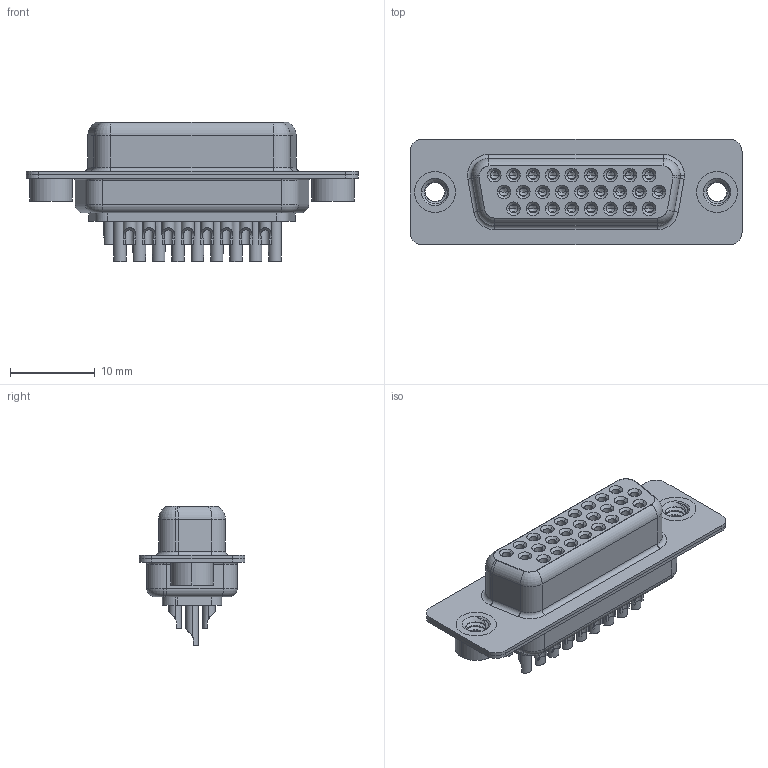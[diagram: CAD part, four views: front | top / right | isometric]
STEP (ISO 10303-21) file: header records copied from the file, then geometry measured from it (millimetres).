
FILE_DESCRIPTION (( 'STEP AP203' ), '1' );
FILE_NAME ('638-M26-332-BN2.STEP', '2022-07-05T19:32:56', ( '' ), ( '' ), 'SwSTEP 2.0', 'SolidWorks 2020', '' );
FILE_SCHEMA (( 'CONFIG_CONTROL_DESIGN' ));
Length unit declared in the file: millimetre
Products named in the file (8): 638M Shell Rear_26 Contacts; 638M Housing_26 Contacts; 638M Contact Row 1_32; 638M Contact Row 3_32; 638-M26-332-BN2; 638M 4-40 Threaded Rivet; 638M Shell Front_26 Contacts; 638M Contact Row 2_32
Assembly tree (31 placements, depth 2):
  638-M26-332-BN2
    638M Housing_26 Contacts
    638M Shell Front_26 Contacts
    638M Shell Rear_26 Contacts
    638M Contact Row 1_32  x9
    638M Contact Row 2_32  x9
    638M Contact Row 3_32  x8
    638M 4-40 Threaded Rivet  x2
Bounding box: 39.2 x 12.5 x 16.45 mm (x, y, z)
Volume: 2392.2 mm3; surface area: 8045.8 mm2
Topology: 31 solids, 31 shells, 1709 faces, 4221 edges, 2611 vertices
Faces by surface type: cylinder 683, plane 509, torus 265, cone 246, bspline 6
Entity records: 23660 total; most frequent: CARTESIAN_POINT 5266, DIRECTION 3880, ORIENTED_EDGE 3288, EDGE_CURVE 1644, AXIS2_PLACEMENT_3D 1626, VERTEX_POINT 1041, CIRCLE 885, EDGE_LOOP 869
